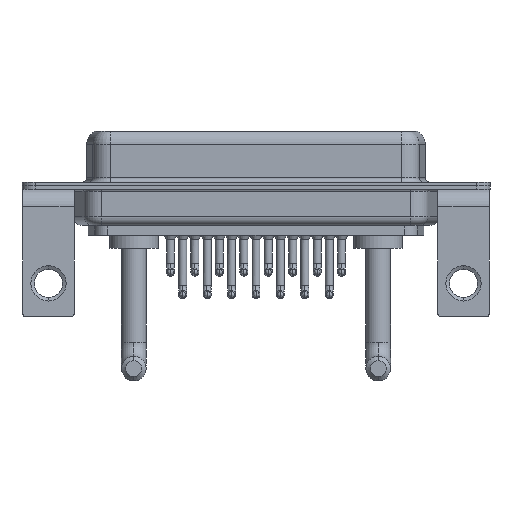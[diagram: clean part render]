
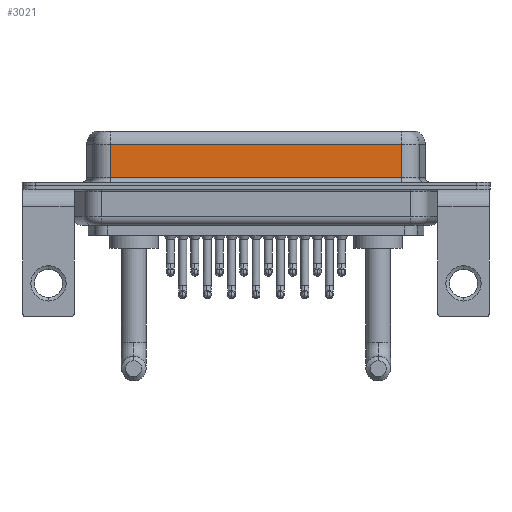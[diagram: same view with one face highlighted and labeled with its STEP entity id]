
A CAD part, front view. The second image highlights one B-rep face of the part: STEP entity #3021.
In plain terms, the highlighted planar face has unit normal (0, -1, 0).
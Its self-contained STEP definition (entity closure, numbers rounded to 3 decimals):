
#244 = VERTEX_POINT ( 'NONE', #2926 ) ;
#1013 = DIRECTION ( 'NONE',  ( 0., 1., 0. ) ) ;
#1210 = VECTOR ( 'NONE', #16566, 1000. ) ;
#1522 = ORIENTED_EDGE ( 'NONE', *, *, #13548, .T. ) ;
#1728 = ORIENTED_EDGE ( 'NONE', *, *, #20143, .F. ) ;
#2215 = LINE ( 'NONE', #3636, #20719 ) ;
#2926 = CARTESIAN_POINT ( 'NONE',  ( 7.013, -3.95, 4.65 ) ) ;
#2954 = VERTEX_POINT ( 'NONE', #9792 ) ;
#3021 = ADVANCED_FACE ( 'NONE', ( #4760 ), #18080, .F. ) ;
#3636 = CARTESIAN_POINT ( 'NONE',  ( 7.013, -3.95, 6.4 ) ) ;
#4086 = DIRECTION ( 'NONE',  ( 0., 0., -1. ) ) ;
#4760 = FACE_OUTER_BOUND ( 'NONE', #18124, .T. ) ;
#5017 = EDGE_CURVE ( 'NONE', #2954, #244, #5503, .T. ) ;
#5503 = LINE ( 'NONE', #15751, #10454 ) ;
#6511 = DIRECTION ( 'NONE',  ( 0., 0., 1. ) ) ;
#8060 = LINE ( 'NONE', #9802, #1210 ) ;
#8152 = CARTESIAN_POINT ( 'NONE',  ( 40.037, -3.95, 6.4 ) ) ;
#9101 = CARTESIAN_POINT ( 'NONE',  ( 40.037, -3.95, 0.9 ) ) ;
#9520 = CARTESIAN_POINT ( 'NONE',  ( 40.037, -3.95, 0.9 ) ) ;
#9792 = CARTESIAN_POINT ( 'NONE',  ( 40.037, -3.95, 4.65 ) ) ;
#9802 = CARTESIAN_POINT ( 'NONE',  ( 40.037, -3.95, 6.4 ) ) ;
#9920 = AXIS2_PLACEMENT_3D ( 'NONE', #8152, #1013, #6511 ) ;
#10332 = VERTEX_POINT ( 'NONE', #17214 ) ;
#10454 = VECTOR ( 'NONE', #12162, 1000. ) ;
#12162 = DIRECTION ( 'NONE',  ( -1., 0., 0. ) ) ;
#12415 = VERTEX_POINT ( 'NONE', #9520 ) ;
#13548 = EDGE_CURVE ( 'NONE', #10332, #12415, #18720, .T. ) ;
#13898 = DIRECTION ( 'NONE',  ( 1., 0., 0. ) ) ;
#15751 = CARTESIAN_POINT ( 'NONE',  ( 40.037, -3.95, 4.65 ) ) ;
#16566 = DIRECTION ( 'NONE',  ( 0., 0., -1. ) ) ;
#16665 = VECTOR ( 'NONE', #13898, 1000. ) ;
#17214 = CARTESIAN_POINT ( 'NONE',  ( 7.013, -3.95, 0.9 ) ) ;
#17306 = ORIENTED_EDGE ( 'NONE', *, *, #18609, .T. ) ;
#18080 = PLANE ( 'NONE',  #9920 ) ;
#18124 = EDGE_LOOP ( 'NONE', ( #1728, #21220, #17306, #1522 ) ) ;
#18609 = EDGE_CURVE ( 'NONE', #244, #10332, #2215, .T. ) ;
#18720 = LINE ( 'NONE', #9101, #16665 ) ;
#20143 = EDGE_CURVE ( 'NONE', #2954, #12415, #8060, .T. ) ;
#20719 = VECTOR ( 'NONE', #4086, 1000. ) ;
#21220 = ORIENTED_EDGE ( 'NONE', *, *, #5017, .T. ) ;
